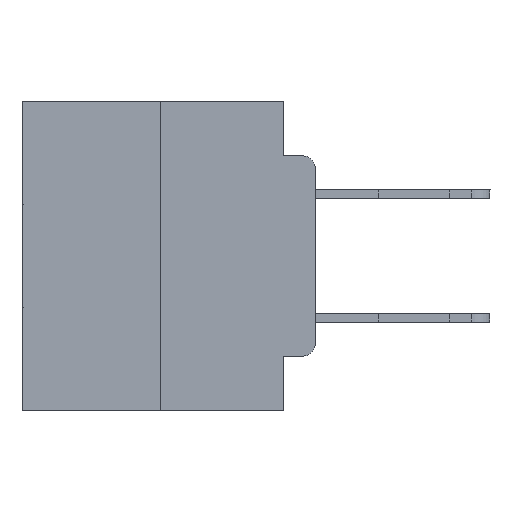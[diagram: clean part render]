
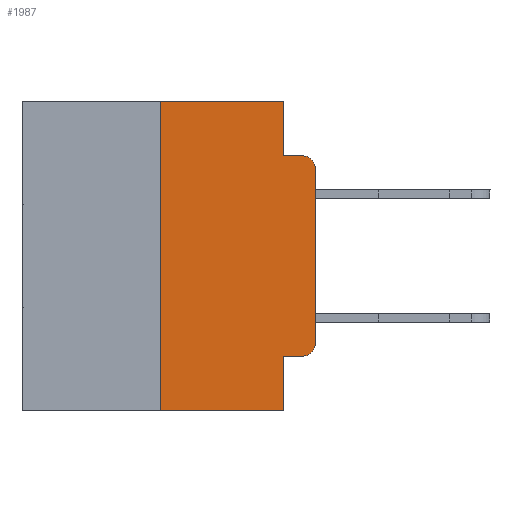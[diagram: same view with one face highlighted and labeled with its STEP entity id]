
A CAD part, left-side view. The second image highlights one B-rep face of the part: STEP entity #1987.
In plain terms, the highlighted planar face has unit normal (-1, 0, 0).
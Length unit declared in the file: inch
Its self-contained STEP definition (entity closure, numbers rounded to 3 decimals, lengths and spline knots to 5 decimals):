
#112 = EDGE_CURVE ( 'NONE', #21272, #25422, #17057, .T. ) ;
#272 = CARTESIAN_POINT ( 'NONE',  ( 0., 0., -0.1085 ) ) ;
#471 = DIRECTION ( 'NONE',  ( 0., 0., -1. ) ) ;
#679 = DIRECTION ( 'NONE',  ( 0., 0., -1. ) ) ;
#899 = VERTEX_POINT ( 'NONE', #16081 ) ;
#1140 = LINE ( 'NONE', #12299, #15764 ) ;
#1321 = CARTESIAN_POINT ( 'NONE',  ( 0., 0.02, -0.4115 ) ) ;
#1368 = CARTESIAN_POINT ( 'NONE',  ( 0., 0.25, 0. ) ) ;
#1788 = CARTESIAN_POINT ( 'NONE',  ( 0., 0.051, -0.4115 ) ) ;
#1878 = DIRECTION ( 'NONE',  ( 0., 0., -1. ) ) ;
#1979 = CARTESIAN_POINT ( 'NONE',  ( 0., 0.051, -0.0885 ) ) ;
#1987 = ADVANCED_FACE ( 'NONE', ( #21348 ), #5355, .F. ) ;
#2027 = AXIS2_PLACEMENT_3D ( 'NONE', #4383, #18012, #15779 ) ;
#2102 = DIRECTION ( 'NONE',  ( -1., 0., 0. ) ) ;
#2314 = ORIENTED_EDGE ( 'NONE', *, *, #27171, .T. ) ;
#3430 = CARTESIAN_POINT ( 'NONE',  ( 0., 0.473, -0.5 ) ) ;
#3724 = DIRECTION ( 'NONE',  ( 0., -1., 0. ) ) ;
#4338 = DIRECTION ( 'NONE',  ( 0., -1., 0. ) ) ;
#4383 = CARTESIAN_POINT ( 'NONE',  ( 0., 0.02, -0.3915 ) ) ;
#5355 = PLANE ( 'NONE',  #22528 ) ;
#5744 = CARTESIAN_POINT ( 'NONE',  ( 0., 0.051, -0.0885 ) ) ;
#6254 = LINE ( 'NONE', #13072, #19739 ) ;
#6266 = ORIENTED_EDGE ( 'NONE', *, *, #13792, .F. ) ;
#6473 = VERTEX_POINT ( 'NONE', #18366 ) ;
#7716 = DIRECTION ( 'NONE',  ( 0., -1., 0. ) ) ;
#7729 = CIRCLE ( 'NONE', #2027, 0.02 ) ;
#8813 = LINE ( 'NONE', #1979, #9417 ) ;
#8912 = DIRECTION ( 'NONE',  ( 0., 0., 1. ) ) ;
#8933 = EDGE_CURVE ( 'NONE', #6473, #21272, #6254, .T. ) ;
#9417 = VECTOR ( 'NONE', #10884, 39.37008 ) ;
#9933 = EDGE_CURVE ( 'NONE', #14113, #25422, #8813, .T. ) ;
#10596 = CARTESIAN_POINT ( 'NONE',  ( 0., 0.02, -0.0885 ) ) ;
#10884 = DIRECTION ( 'NONE',  ( 0., -1., 0. ) ) ;
#11375 = ORIENTED_EDGE ( 'NONE', *, *, #22710, .F. ) ;
#11683 = CARTESIAN_POINT ( 'NONE',  ( 0., 0.051, -0.5 ) ) ;
#11970 = VERTEX_POINT ( 'NONE', #1321 ) ;
#12299 = CARTESIAN_POINT ( 'NONE',  ( 0., 0.473, 0. ) ) ;
#12327 = LINE ( 'NONE', #3430, #12861 ) ;
#12685 = CARTESIAN_POINT ( 'NONE',  ( 0., 0.051, 0. ) ) ;
#12861 = VECTOR ( 'NONE', #3724, 39.37008 ) ;
#12897 = CARTESIAN_POINT ( 'NONE',  ( 0., 0.25, 0. ) ) ;
#13072 = CARTESIAN_POINT ( 'NONE',  ( 0., 0., 0. ) ) ;
#13518 = CARTESIAN_POINT ( 'NONE',  ( 0., 0.02, -0.1085 ) ) ;
#13792 = EDGE_CURVE ( 'NONE', #25311, #14113, #19413, .T. ) ;
#14026 = EDGE_CURVE ( 'NONE', #23303, #18429, #21463, .T. ) ;
#14081 = DIRECTION ( 'NONE',  ( 1., 0., 0. ) ) ;
#14113 = VERTEX_POINT ( 'NONE', #5744 ) ;
#14606 = VERTEX_POINT ( 'NONE', #1368 ) ;
#14680 = AXIS2_PLACEMENT_3D ( 'NONE', #13518, #2102, #471 ) ;
#14969 = EDGE_LOOP ( 'NONE', ( #23779, #22265, #22458, #6266, #11375, #27252, #28943, #27675, #2314, #23179 ) ) ;
#15239 = EDGE_CURVE ( 'NONE', #899, #14606, #21814, .T. ) ;
#15764 = VECTOR ( 'NONE', #7716, 39.37008 ) ;
#15779 = DIRECTION ( 'NONE',  ( 0., 0., -1. ) ) ;
#16081 = CARTESIAN_POINT ( 'NONE',  ( 0., 0.25, -0.5 ) ) ;
#16535 = VECTOR ( 'NONE', #679, 39.37008 ) ;
#17057 = CIRCLE ( 'NONE', #14680, 0.02 ) ;
#17497 = VECTOR ( 'NONE', #1878, 39.37008 ) ;
#17668 = LINE ( 'NONE', #1788, #21617 ) ;
#18012 = DIRECTION ( 'NONE',  ( -1., 0., 0. ) ) ;
#18366 = CARTESIAN_POINT ( 'NONE',  ( 0., 0., -0.3915 ) ) ;
#18429 = VERTEX_POINT ( 'NONE', #11683 ) ;
#18515 = CARTESIAN_POINT ( 'NONE',  ( 0., 0.051, 0. ) ) ;
#19413 = LINE ( 'NONE', #28767, #17497 ) ;
#19739 = VECTOR ( 'NONE', #8912, 39.37008 ) ;
#20897 = CARTESIAN_POINT ( 'NONE',  ( 0., 0.051, -0.4115 ) ) ;
#21045 = EDGE_CURVE ( 'NONE', #899, #18429, #12327, .T. ) ;
#21211 = CARTESIAN_POINT ( 'NONE',  ( 0., 0.473, 0. ) ) ;
#21272 = VERTEX_POINT ( 'NONE', #272 ) ;
#21348 = FACE_OUTER_BOUND ( 'NONE', #14969, .T. ) ;
#21463 = LINE ( 'NONE', #18515, #16535 ) ;
#21617 = VECTOR ( 'NONE', #4338, 39.37008 ) ;
#21814 = LINE ( 'NONE', #12897, #22170 ) ;
#22105 = DIRECTION ( 'NONE',  ( 0., 0., 1. ) ) ;
#22170 = VECTOR ( 'NONE', #22105, 39.37008 ) ;
#22182 = EDGE_CURVE ( 'NONE', #11970, #6473, #7729, .T. ) ;
#22265 = ORIENTED_EDGE ( 'NONE', *, *, #112, .T. ) ;
#22458 = ORIENTED_EDGE ( 'NONE', *, *, #9933, .F. ) ;
#22528 = AXIS2_PLACEMENT_3D ( 'NONE', #21211, #14081, #25959 ) ;
#22710 = EDGE_CURVE ( 'NONE', #14606, #25311, #1140, .T. ) ;
#23179 = ORIENTED_EDGE ( 'NONE', *, *, #22182, .T. ) ;
#23303 = VERTEX_POINT ( 'NONE', #20897 ) ;
#23779 = ORIENTED_EDGE ( 'NONE', *, *, #8933, .T. ) ;
#25311 = VERTEX_POINT ( 'NONE', #12685 ) ;
#25422 = VERTEX_POINT ( 'NONE', #10596 ) ;
#25959 = DIRECTION ( 'NONE',  ( 0., 0., -1. ) ) ;
#27171 = EDGE_CURVE ( 'NONE', #23303, #11970, #17668, .T. ) ;
#27252 = ORIENTED_EDGE ( 'NONE', *, *, #15239, .F. ) ;
#27675 = ORIENTED_EDGE ( 'NONE', *, *, #14026, .F. ) ;
#28767 = CARTESIAN_POINT ( 'NONE',  ( 0., 0.051, 0. ) ) ;
#28943 = ORIENTED_EDGE ( 'NONE', *, *, #21045, .T. ) ;
